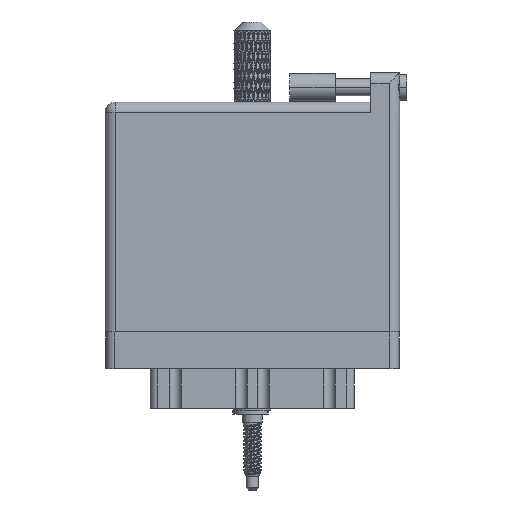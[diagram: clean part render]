
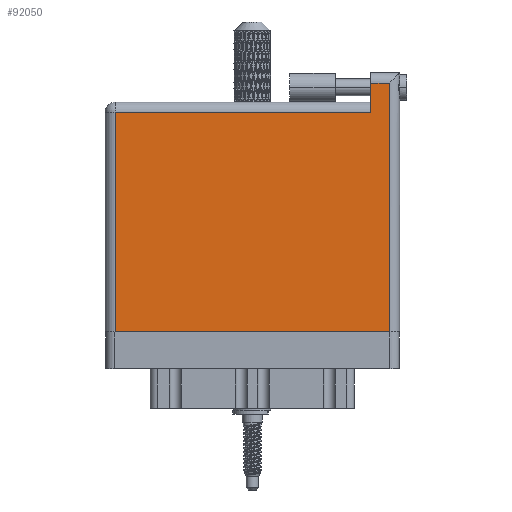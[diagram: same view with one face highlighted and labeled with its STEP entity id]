
A CAD part, front view. The second image highlights one B-rep face of the part: STEP entity #92050.
In plain terms, the highlighted face is planar.
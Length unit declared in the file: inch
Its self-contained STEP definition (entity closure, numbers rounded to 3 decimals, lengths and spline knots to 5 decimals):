
#323 = DIRECTION ( 'NONE',  ( 0., 0., -1. ) ) ;
#2292 = VERTEX_POINT ( 'NONE', #71920 ) ;
#15204 = CARTESIAN_POINT ( 'NONE',  ( 1.811, 1.696, 0. ) ) ;
#16153 = DIRECTION ( 'NONE',  ( -1., 0., 0. ) ) ;
#17905 = DIRECTION ( 'NONE',  ( -1., 0., 0. ) ) ;
#19569 = ORIENTED_EDGE ( 'NONE', *, *, #90755, .T. ) ;
#21965 = CARTESIAN_POINT ( 'NONE',  ( 0., 0., 0. ) ) ;
#23419 = LINE ( 'NONE', #87735, #72491 ) ;
#26224 = EDGE_CURVE ( 'NONE', #2292, #56328, #61036, .T. ) ;
#26351 = CARTESIAN_POINT ( 'NONE',  ( 0.07, 1.496, 0. ) ) ;
#26503 = CARTESIAN_POINT ( 'NONE',  ( 1.938, 1.766, 0. ) ) ;
#26918 = EDGE_CURVE ( 'NONE', #36168, #2292, #50792, .T. ) ;
#28563 = DIRECTION ( 'NONE',  ( 0., 1., 0. ) ) ;
#31459 = FACE_OUTER_BOUND ( 'NONE', #70997, .T. ) ;
#32956 = ORIENTED_EDGE ( 'NONE', *, *, #26224, .T. ) ;
#33406 = CARTESIAN_POINT ( 'NONE',  ( 0.07, 0., 0. ) ) ;
#34140 = ORIENTED_EDGE ( 'NONE', *, *, #36844, .T. ) ;
#35474 = LINE ( 'NONE', #26503, #62612 ) ;
#36168 = VERTEX_POINT ( 'NONE', #26351 ) ;
#36844 = EDGE_CURVE ( 'NONE', #77034, #64014, #73811, .T. ) ;
#43763 = LINE ( 'NONE', #74846, #52986 ) ;
#46917 = CARTESIAN_POINT ( 'NONE',  ( 1.938, 1.696, 0. ) ) ;
#49195 = AXIS2_PLACEMENT_3D ( 'NONE', #55744, #323, #16153 ) ;
#50792 = LINE ( 'NONE', #33406, #91541 ) ;
#52986 = VECTOR ( 'NONE', #75888, 39.37008 ) ;
#53544 = EDGE_CURVE ( 'NONE', #58318, #36168, #43763, .T. ) ;
#55744 = CARTESIAN_POINT ( 'NONE',  ( 0., 1.566, 0. ) ) ;
#56328 = VERTEX_POINT ( 'NONE', #87145 ) ;
#58318 = VERTEX_POINT ( 'NONE', #86605 ) ;
#59757 = DIRECTION ( 'NONE',  ( 0., -1., 0. ) ) ;
#61036 = LINE ( 'NONE', #21965, #71318 ) ;
#62612 = VECTOR ( 'NONE', #28563, 39.37008 ) ;
#64014 = VERTEX_POINT ( 'NONE', #15204 ) ;
#64701 = PLANE ( 'NONE',  #49195 ) ;
#66049 = VECTOR ( 'NONE', #17905, 39.37008 ) ;
#67034 = ORIENTED_EDGE ( 'NONE', *, *, #53544, .T. ) ;
#69900 = ORIENTED_EDGE ( 'NONE', *, *, #72021, .T. ) ;
#70997 = EDGE_LOOP ( 'NONE', ( #32956, #19569, #34140, #69900, #67034, #78516 ) ) ;
#71318 = VECTOR ( 'NONE', #86795, 39.37008 ) ;
#71920 = CARTESIAN_POINT ( 'NONE',  ( 0.07, 0., 0. ) ) ;
#72021 = EDGE_CURVE ( 'NONE', #64014, #58318, #23419, .T. ) ;
#72491 = VECTOR ( 'NONE', #94045, 39.37008 ) ;
#73811 = LINE ( 'NONE', #99087, #66049 ) ;
#74846 = CARTESIAN_POINT ( 'NONE',  ( 0., 1.496, 0. ) ) ;
#75888 = DIRECTION ( 'NONE',  ( -1., 0., 0. ) ) ;
#77034 = VERTEX_POINT ( 'NONE', #46917 ) ;
#78516 = ORIENTED_EDGE ( 'NONE', *, *, #26918, .T. ) ;
#86605 = CARTESIAN_POINT ( 'NONE',  ( 1.811, 1.496, 0. ) ) ;
#86795 = DIRECTION ( 'NONE',  ( 1., 0., 0. ) ) ;
#87145 = CARTESIAN_POINT ( 'NONE',  ( 1.938, 0., 0. ) ) ;
#87735 = CARTESIAN_POINT ( 'NONE',  ( 1.811, 1.766, 0. ) ) ;
#90755 = EDGE_CURVE ( 'NONE', #56328, #77034, #35474, .T. ) ;
#91541 = VECTOR ( 'NONE', #59757, 39.37008 ) ;
#92050 = ADVANCED_FACE ( 'NONE', ( #31459 ), #64701, .F. ) ;
#94045 = DIRECTION ( 'NONE',  ( 0., -1., 0. ) ) ;
#99087 = CARTESIAN_POINT ( 'NONE',  ( 0., 1.696, 0. ) ) ;
